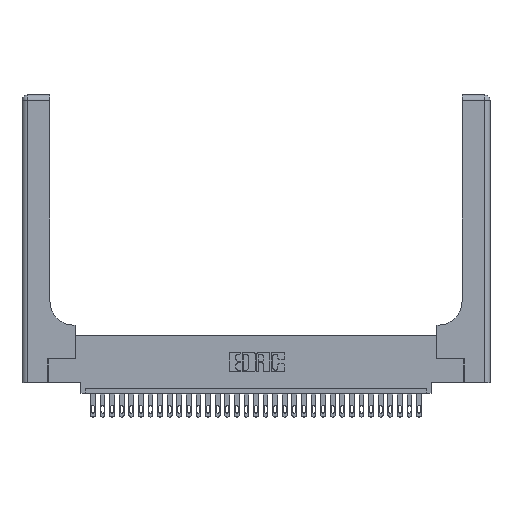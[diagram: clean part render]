
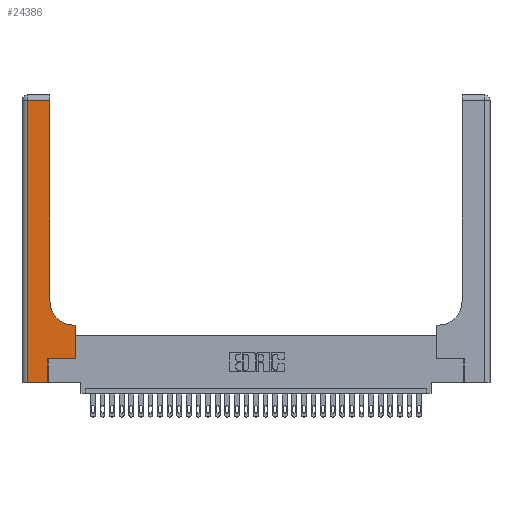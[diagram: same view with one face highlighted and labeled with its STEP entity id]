
A CAD part, top view. The second image highlights one B-rep face of the part: STEP entity #24386.
In plain terms, the highlighted planar face has unit normal (0, 0, 1).
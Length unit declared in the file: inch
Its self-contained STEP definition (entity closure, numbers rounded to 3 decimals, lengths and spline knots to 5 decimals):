
#163 = ORIENTED_EDGE ( 'NONE', *, *, #19725, .T. ) ;
#1690 = EDGE_CURVE ( 'NONE', #19468, #6464, #13135, .T. ) ;
#1806 = AXIS2_PLACEMENT_3D ( 'NONE', #27033, #29561, #22295 ) ;
#2808 = DIRECTION ( 'NONE',  ( 0., 1., 0. ) ) ;
#3007 = DIRECTION ( 'NONE',  ( 1., 0., 0. ) ) ;
#3122 = EDGE_CURVE ( 'NONE', #20000, #12582, #4371, .T. ) ;
#4371 = CIRCLE ( 'NONE', #1806, 0.25 ) ;
#4480 = CARTESIAN_POINT ( 'NONE',  ( 0.269, 0., 0.37 ) ) ;
#6464 = VERTEX_POINT ( 'NONE', #29768 ) ;
#6850 = DIRECTION ( 'NONE',  ( 0., 1., 0. ) ) ;
#6921 = EDGE_CURVE ( 'NONE', #19274, #20000, #14997, .T. ) ;
#7209 = CARTESIAN_POINT ( 'NONE',  ( 0.2915, 2.94, 0.37 ) ) ;
#7799 = LINE ( 'NONE', #18173, #15339 ) ;
#7888 = VERTEX_POINT ( 'NONE', #13175 ) ;
#8238 = VECTOR ( 'NONE', #28826, 39.37008 ) ;
#8263 = LINE ( 'NONE', #10342, #9868 ) ;
#8369 = FACE_OUTER_BOUND ( 'NONE', #25866, .T. ) ;
#8651 = CARTESIAN_POINT ( 'NONE',  ( 0.2915, 0.85, 0.37 ) ) ;
#9182 = VECTOR ( 'NONE', #2808, 39.37008 ) ;
#9313 = AXIS2_PLACEMENT_3D ( 'NONE', #27735, #27535, #12743 ) ;
#9868 = VECTOR ( 'NONE', #30294, 39.37008 ) ;
#10170 = CARTESIAN_POINT ( 'NONE',  ( 0., 0., 0.37 ) ) ;
#10192 = PLANE ( 'NONE',  #9313 ) ;
#10342 = CARTESIAN_POINT ( 'NONE',  ( 0.06, 3., 0.37 ) ) ;
#10389 = ORIENTED_EDGE ( 'NONE', *, *, #1690, .T. ) ;
#11887 = VERTEX_POINT ( 'NONE', #14088 ) ;
#12582 = VERTEX_POINT ( 'NONE', #8651 ) ;
#12743 = DIRECTION ( 'NONE',  ( -1., 0., 0. ) ) ;
#13004 = VECTOR ( 'NONE', #23950, 39.37008 ) ;
#13135 = LINE ( 'NONE', #25241, #9182 ) ;
#13175 = CARTESIAN_POINT ( 'NONE',  ( 0.06, 0., 0.37 ) ) ;
#14088 = CARTESIAN_POINT ( 'NONE',  ( 0.5585, 0.25, 0.37 ) ) ;
#14997 = LINE ( 'NONE', #23504, #8238 ) ;
#15339 = VECTOR ( 'NONE', #3007, 39.37008 ) ;
#17746 = ORIENTED_EDGE ( 'NONE', *, *, #3122, .T. ) ;
#17783 = EDGE_CURVE ( 'NONE', #11887, #19274, #31651, .T. ) ;
#18173 = CARTESIAN_POINT ( 'NONE',  ( 0.269, 0.25, 0.37 ) ) ;
#18465 = ORIENTED_EDGE ( 'NONE', *, *, #6921, .T. ) ;
#19141 = CARTESIAN_POINT ( 'NONE',  ( 0.06, 2.94, 0.37 ) ) ;
#19274 = VERTEX_POINT ( 'NONE', #29076 ) ;
#19468 = VERTEX_POINT ( 'NONE', #4480 ) ;
#19725 = EDGE_CURVE ( 'NONE', #7888, #19468, #31527, .T. ) ;
#20000 = VERTEX_POINT ( 'NONE', #29790 ) ;
#20291 = VECTOR ( 'NONE', #28311, 39.37008 ) ;
#21259 = EDGE_CURVE ( 'NONE', #12582, #32482, #28267, .T. ) ;
#21869 = CARTESIAN_POINT ( 'NONE',  ( 0.2915, 3., 0.37 ) ) ;
#22295 = DIRECTION ( 'NONE',  ( 1., 0., 0. ) ) ;
#23504 = CARTESIAN_POINT ( 'NONE',  ( 0.2915, 0.6, 0.37 ) ) ;
#23521 = LINE ( 'NONE', #24180, #13004 ) ;
#23950 = DIRECTION ( 'NONE',  ( -1., 0., 0. ) ) ;
#24028 = VECTOR ( 'NONE', #26159, 39.37008 ) ;
#24180 = CARTESIAN_POINT ( 'NONE',  ( 0., 2.94, 0.37 ) ) ;
#24386 = ADVANCED_FACE ( 'NONE', ( #8369 ), #10192, .F. ) ;
#25119 = ORIENTED_EDGE ( 'NONE', *, *, #21259, .T. ) ;
#25241 = CARTESIAN_POINT ( 'NONE',  ( 0.269, 0., 0.37 ) ) ;
#25314 = VERTEX_POINT ( 'NONE', #19141 ) ;
#25320 = CARTESIAN_POINT ( 'NONE',  ( 0.5585, 0.25, 0.37 ) ) ;
#25866 = EDGE_LOOP ( 'NONE', ( #25119, #31314, #32051, #163, #10389, #28752, #28113, #18465, #17746 ) ) ;
#26159 = DIRECTION ( 'NONE',  ( 1., 0., 0. ) ) ;
#26426 = EDGE_CURVE ( 'NONE', #32482, #25314, #23521, .T. ) ;
#26697 = EDGE_CURVE ( 'NONE', #25314, #7888, #8263, .T. ) ;
#27033 = CARTESIAN_POINT ( 'NONE',  ( 0.5415, 0.85, 0.37 ) ) ;
#27535 = DIRECTION ( 'NONE',  ( 0., 0., -1. ) ) ;
#27735 = CARTESIAN_POINT ( 'NONE',  ( 0., 3., 0.37 ) ) ;
#28113 = ORIENTED_EDGE ( 'NONE', *, *, #17783, .T. ) ;
#28267 = LINE ( 'NONE', #21869, #31414 ) ;
#28311 = DIRECTION ( 'NONE',  ( 0., 1., 0. ) ) ;
#28752 = ORIENTED_EDGE ( 'NONE', *, *, #29693, .T. ) ;
#28826 = DIRECTION ( 'NONE',  ( -1., 0., 0. ) ) ;
#29076 = CARTESIAN_POINT ( 'NONE',  ( 0.5585, 0.6, 0.37 ) ) ;
#29561 = DIRECTION ( 'NONE',  ( 0., 0., -1. ) ) ;
#29693 = EDGE_CURVE ( 'NONE', #6464, #11887, #7799, .T. ) ;
#29768 = CARTESIAN_POINT ( 'NONE',  ( 0.269, 0.25, 0.37 ) ) ;
#29790 = CARTESIAN_POINT ( 'NONE',  ( 0.5415, 0.6, 0.37 ) ) ;
#30294 = DIRECTION ( 'NONE',  ( 0., -1., 0. ) ) ;
#31314 = ORIENTED_EDGE ( 'NONE', *, *, #26426, .T. ) ;
#31414 = VECTOR ( 'NONE', #6850, 39.37008 ) ;
#31527 = LINE ( 'NONE', #10170, #24028 ) ;
#31651 = LINE ( 'NONE', #25320, #20291 ) ;
#32051 = ORIENTED_EDGE ( 'NONE', *, *, #26697, .T. ) ;
#32482 = VERTEX_POINT ( 'NONE', #7209 ) ;
